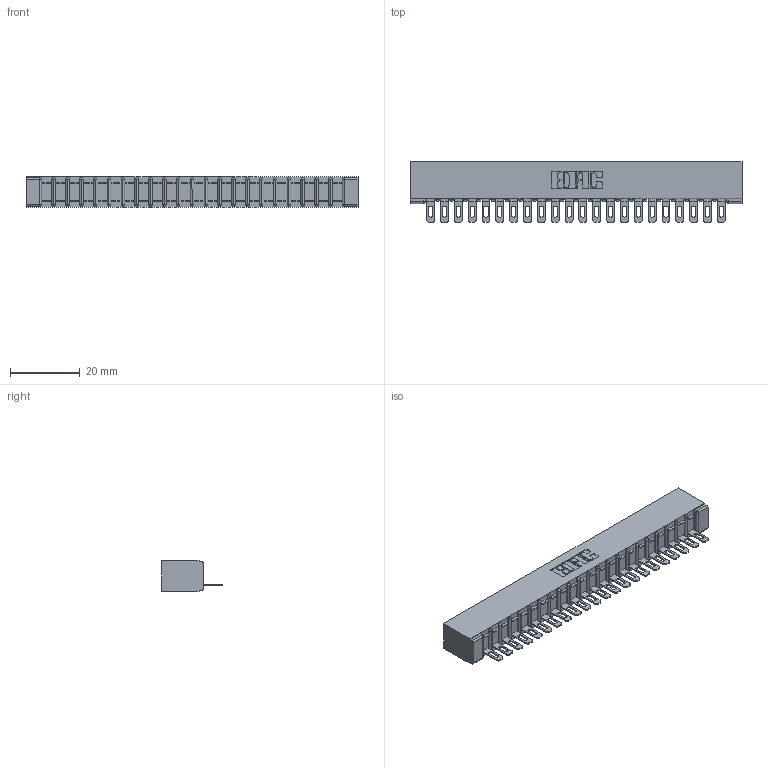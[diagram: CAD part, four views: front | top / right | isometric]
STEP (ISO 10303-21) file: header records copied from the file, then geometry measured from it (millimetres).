
FILE_DESCRIPTION (( 'STEP AP203' ), '1' );
FILE_NAME ('307-022-401-101.STEP', '2020-09-27T06:32:27', ( '' ), ( '' ), 'SwSTEP 2.0', 'SolidWorks 2020', '' );
FILE_SCHEMA (( 'CONFIG_CONTROL_DESIGN' ));
Length unit declared in the file: inch
Products named in the file (3): 307 Part_No Mounting Lugs; 307-290-002_501; 307-022-401-101
Assembly tree (23 placements, depth 2):
  307-022-401-101
    307 Part_No Mounting Lugs
    307-290-002_501  x22
Bounding box: 95.05 x 17.42 x 8.71 mm (x, y, z)
Volume: 6536.3 mm3; surface area: 12543.7 mm2
Topology: 23 solids, 23 shells, 1805 faces, 5535 edges, 3626 vertices
Faces by surface type: plane 1034, cylinder 725, sphere 46
Entity records: 21842 total; most frequent: CARTESIAN_POINT 3680, ORIENTED_EDGE 3670, DIRECTION 3587, EDGE_CURVE 1835, LINE 1393, VECTOR 1393, VERTEX_POINT 1190, AXIS2_PLACEMENT_3D 1097
